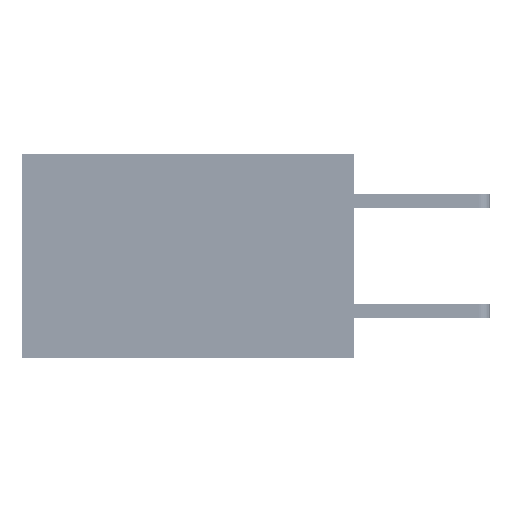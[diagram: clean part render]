
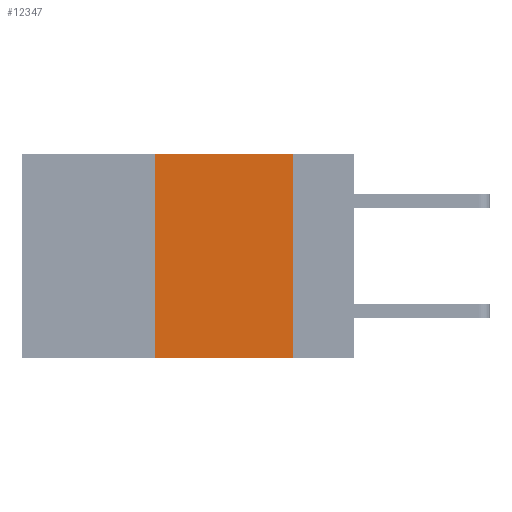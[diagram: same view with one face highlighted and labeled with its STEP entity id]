
A CAD part, left-side view. The second image highlights one B-rep face of the part: STEP entity #12347.
In plain terms, the highlighted planar face has unit normal (-1, 0, 0).
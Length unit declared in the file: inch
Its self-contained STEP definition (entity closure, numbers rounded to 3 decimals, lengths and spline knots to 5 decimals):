
#1344 = VERTEX_POINT ( 'NONE', #8260 ) ;
#4273 = DIRECTION ( 'NONE',  ( 0., -1., 0. ) ) ;
#4507 = CARTESIAN_POINT ( 'NONE',  ( 0., 0.6, 0. ) ) ;
#6441 = DIRECTION ( 'NONE',  ( 0., -1., 0. ) ) ;
#6816 = CARTESIAN_POINT ( 'NONE',  ( 0., 0.36, -0.37 ) ) ;
#7078 = ORIENTED_EDGE ( 'NONE', *, *, #13955, .F. ) ;
#8260 = CARTESIAN_POINT ( 'NONE',  ( 0., 0.11, 0. ) ) ;
#9051 = ORIENTED_EDGE ( 'NONE', *, *, #22932, .F. ) ;
#9302 = EDGE_CURVE ( 'NONE', #1344, #25480, #21158, .T. ) ;
#9806 = LINE ( 'NONE', #33925, #10399 ) ;
#10344 = VECTOR ( 'NONE', #4273, 39.37008 ) ;
#10399 = VECTOR ( 'NONE', #6441, 39.37008 ) ;
#10811 = VECTOR ( 'NONE', #39493, 39.37008 ) ;
#12347 = ADVANCED_FACE ( 'NONE', ( #38319 ), #38100, .F. ) ;
#13742 = DIRECTION ( 'NONE',  ( 0., 0., -1. ) ) ;
#13955 = EDGE_CURVE ( 'NONE', #19259, #40029, #18767, .T. ) ;
#18767 = LINE ( 'NONE', #21915, #10811 ) ;
#19259 = VERTEX_POINT ( 'NONE', #6816 ) ;
#20763 = CARTESIAN_POINT ( 'NONE',  ( 0., 0.36, 0. ) ) ;
#21158 = LINE ( 'NONE', #34883, #30054 ) ;
#21652 = DIRECTION ( 'NONE',  ( 1., 0., 0. ) ) ;
#21915 = CARTESIAN_POINT ( 'NONE',  ( 0., 0.36, 0. ) ) ;
#22635 = EDGE_LOOP ( 'NONE', ( #32864, #9051, #7078, #32726 ) ) ;
#22932 = EDGE_CURVE ( 'NONE', #40029, #1344, #27690, .T. ) ;
#23746 = EDGE_CURVE ( 'NONE', #19259, #25480, #9806, .T. ) ;
#25480 = VERTEX_POINT ( 'NONE', #26098 ) ;
#26098 = CARTESIAN_POINT ( 'NONE',  ( 0., 0.11, -0.37 ) ) ;
#27690 = LINE ( 'NONE', #31312, #10344 ) ;
#30054 = VECTOR ( 'NONE', #13742, 39.37008 ) ;
#30860 = AXIS2_PLACEMENT_3D ( 'NONE', #4507, #21652, #38775 ) ;
#31312 = CARTESIAN_POINT ( 'NONE',  ( 0., 0.6, 0. ) ) ;
#32726 = ORIENTED_EDGE ( 'NONE', *, *, #23746, .T. ) ;
#32864 = ORIENTED_EDGE ( 'NONE', *, *, #9302, .F. ) ;
#33925 = CARTESIAN_POINT ( 'NONE',  ( 0., 0.6, -0.37 ) ) ;
#34883 = CARTESIAN_POINT ( 'NONE',  ( 0., 0.11, 0. ) ) ;
#38100 = PLANE ( 'NONE',  #30860 ) ;
#38319 = FACE_OUTER_BOUND ( 'NONE', #22635, .T. ) ;
#38775 = DIRECTION ( 'NONE',  ( 0., 0., -1. ) ) ;
#39493 = DIRECTION ( 'NONE',  ( 0., 0., 1. ) ) ;
#40029 = VERTEX_POINT ( 'NONE', #20763 ) ;
